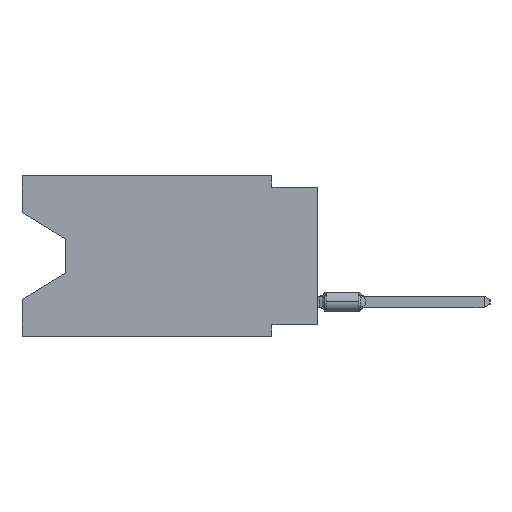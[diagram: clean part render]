
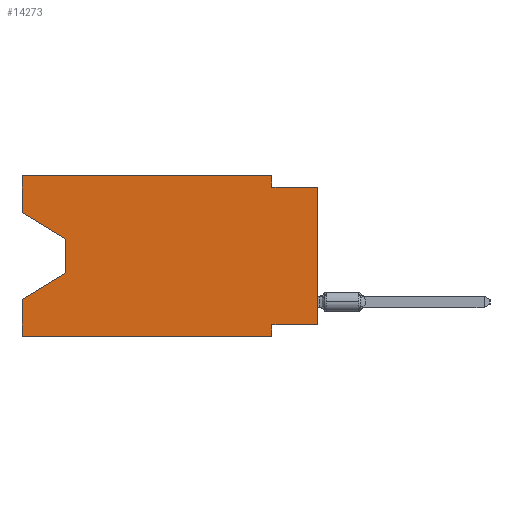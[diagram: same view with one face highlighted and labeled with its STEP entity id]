
A CAD part, left-side view. The second image highlights one B-rep face of the part: STEP entity #14273.
In plain terms, the highlighted planar face has unit normal (-1, 0, 0).
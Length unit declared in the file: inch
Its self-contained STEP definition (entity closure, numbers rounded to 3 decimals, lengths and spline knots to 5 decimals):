
#684 = CARTESIAN_POINT ( 'NONE',  ( 0., 0.645, 0. ) ) ;
#701 = VECTOR ( 'NONE', #1604, 39.37008 ) ;
#1151 = LINE ( 'NONE', #12964, #7756 ) ;
#1463 = EDGE_CURVE ( 'NONE', #5484, #10163, #1151, .T. ) ;
#1604 = DIRECTION ( 'NONE',  ( 0., -1., 0. ) ) ;
#1770 = ORIENTED_EDGE ( 'NONE', *, *, #31686, .F. ) ;
#1779 = DIRECTION ( 'NONE',  ( 0., 0., -1. ) ) ;
#1831 = VERTEX_POINT ( 'NONE', #27846 ) ;
#1860 = FACE_OUTER_BOUND ( 'NONE', #2146, .T. ) ;
#2146 = EDGE_LOOP ( 'NONE', ( #7683, #23044, #23969, #3546, #34981, #1770, #17881, #25467, #27261, #25746, #18919, #8743 ) ) ;
#2795 = VECTOR ( 'NONE', #15203, 39.37008 ) ;
#3060 = VERTEX_POINT ( 'NONE', #7651 ) ;
#3546 = ORIENTED_EDGE ( 'NONE', *, *, #9746, .F. ) ;
#3552 = CARTESIAN_POINT ( 'NONE',  ( 0., 0., -0.325 ) ) ;
#4150 = CARTESIAN_POINT ( 'NONE',  ( 0., 0.55, -0.138 ) ) ;
#4724 = CARTESIAN_POINT ( 'NONE',  ( 0., 0.645, -0.08025 ) ) ;
#5278 = CARTESIAN_POINT ( 'NONE',  ( 0., 0.1, 0. ) ) ;
#5484 = VERTEX_POINT ( 'NONE', #6493 ) ;
#6407 = EDGE_CURVE ( 'NONE', #21673, #17458, #6776, .T. ) ;
#6493 = CARTESIAN_POINT ( 'NONE',  ( 0., 0.645, 0. ) ) ;
#6745 = CARTESIAN_POINT ( 'NONE',  ( 0., 0.1, -0.35 ) ) ;
#6776 = LINE ( 'NONE', #18377, #36574 ) ;
#7187 = LINE ( 'NONE', #34100, #22652 ) ;
#7419 = CARTESIAN_POINT ( 'NONE',  ( 0., 0., -0.025 ) ) ;
#7461 = VERTEX_POINT ( 'NONE', #4724 ) ;
#7474 = PLANE ( 'NONE',  #12363 ) ;
#7651 = CARTESIAN_POINT ( 'NONE',  ( 0., 0.645, -0.35 ) ) ;
#7683 = ORIENTED_EDGE ( 'NONE', *, *, #23505, .T. ) ;
#7756 = VECTOR ( 'NONE', #36549, 39.37008 ) ;
#8116 = CARTESIAN_POINT ( 'NONE',  ( 0., 0.55, -0.138 ) ) ;
#8607 = VERTEX_POINT ( 'NONE', #4150 ) ;
#8667 = EDGE_CURVE ( 'NONE', #3060, #23966, #19072, .T. ) ;
#8743 = ORIENTED_EDGE ( 'NONE', *, *, #22856, .F. ) ;
#9105 = VECTOR ( 'NONE', #21374, 39.37008 ) ;
#9387 = DIRECTION ( 'NONE',  ( 0., 0., 1. ) ) ;
#9746 = EDGE_CURVE ( 'NONE', #3060, #17458, #10046, .T. ) ;
#10046 = LINE ( 'NONE', #21852, #18898 ) ;
#10163 = VERTEX_POINT ( 'NONE', #5278 ) ;
#10171 = DIRECTION ( 'NONE',  ( 1., 0., 0. ) ) ;
#11405 = LINE ( 'NONE', #8116, #35694 ) ;
#12300 = LINE ( 'NONE', #684, #28951 ) ;
#12363 = AXIS2_PLACEMENT_3D ( 'NONE', #19284, #10171, #13275 ) ;
#12964 = CARTESIAN_POINT ( 'NONE',  ( 0., 0.645, 0. ) ) ;
#13275 = DIRECTION ( 'NONE',  ( 0., 0., -1. ) ) ;
#13342 = DIRECTION ( 'NONE',  ( 0., -0.855, -0.519 ) ) ;
#13909 = LINE ( 'NONE', #16812, #34516 ) ;
#14273 = ADVANCED_FACE ( 'NONE', ( #1860 ), #7474, .F. ) ;
#14809 = LINE ( 'NONE', #24293, #31483 ) ;
#15203 = DIRECTION ( 'NONE',  ( 0., -1., 0. ) ) ;
#15305 = CARTESIAN_POINT ( 'NONE',  ( 0., 0.645, -0.26975 ) ) ;
#16230 = CARTESIAN_POINT ( 'NONE',  ( 0., 0., -0.025 ) ) ;
#16812 = CARTESIAN_POINT ( 'NONE',  ( 0., 0.645, -0.08025 ) ) ;
#17161 = EDGE_CURVE ( 'NONE', #1831, #17976, #27742, .T. ) ;
#17403 = CARTESIAN_POINT ( 'NONE',  ( 0., 0.55, -0.212 ) ) ;
#17458 = VERTEX_POINT ( 'NONE', #15305 ) ;
#17881 = ORIENTED_EDGE ( 'NONE', *, *, #35083, .F. ) ;
#17976 = VERTEX_POINT ( 'NONE', #16230 ) ;
#18377 = CARTESIAN_POINT ( 'NONE',  ( 0., 0.55, -0.212 ) ) ;
#18898 = VECTOR ( 'NONE', #33636, 39.37008 ) ;
#18919 = ORIENTED_EDGE ( 'NONE', *, *, #1463, .F. ) ;
#19072 = LINE ( 'NONE', #30870, #2795 ) ;
#19284 = CARTESIAN_POINT ( 'NONE',  ( 0., 0.645, 0. ) ) ;
#20554 = VERTEX_POINT ( 'NONE', #32668 ) ;
#21374 = DIRECTION ( 'NONE',  ( 0., 1., 0. ) ) ;
#21673 = VERTEX_POINT ( 'NONE', #17403 ) ;
#21852 = CARTESIAN_POINT ( 'NONE',  ( 0., 0.645, 0. ) ) ;
#22652 = VECTOR ( 'NONE', #1779, 39.37008 ) ;
#22856 = EDGE_CURVE ( 'NONE', #7461, #5484, #12300, .T. ) ;
#23044 = ORIENTED_EDGE ( 'NONE', *, *, #33446, .T. ) ;
#23505 = EDGE_CURVE ( 'NONE', #7461, #8607, #13909, .T. ) ;
#23921 = DIRECTION ( 'NONE',  ( 0., 0., 1. ) ) ;
#23966 = VERTEX_POINT ( 'NONE', #6745 ) ;
#23969 = ORIENTED_EDGE ( 'NONE', *, *, #6407, .T. ) ;
#24293 = CARTESIAN_POINT ( 'NONE',  ( 0., 0., 0. ) ) ;
#25467 = ORIENTED_EDGE ( 'NONE', *, *, #37052, .T. ) ;
#25746 = ORIENTED_EDGE ( 'NONE', *, *, #30778, .F. ) ;
#27261 = ORIENTED_EDGE ( 'NONE', *, *, #17161, .F. ) ;
#27742 = LINE ( 'NONE', #7419, #701 ) ;
#27846 = CARTESIAN_POINT ( 'NONE',  ( 0., 0.1, -0.025 ) ) ;
#28951 = VECTOR ( 'NONE', #23921, 39.37008 ) ;
#29361 = LINE ( 'NONE', #34961, #29796 ) ;
#29796 = VECTOR ( 'NONE', #38240, 39.37008 ) ;
#30778 = EDGE_CURVE ( 'NONE', #10163, #1831, #29361, .T. ) ;
#30870 = CARTESIAN_POINT ( 'NONE',  ( 0., 0.645, -0.35 ) ) ;
#31483 = VECTOR ( 'NONE', #9387, 39.37008 ) ;
#31686 = EDGE_CURVE ( 'NONE', #20554, #23966, #7187, .T. ) ;
#32668 = CARTESIAN_POINT ( 'NONE',  ( 0., 0.1, -0.325 ) ) ;
#33165 = LINE ( 'NONE', #3552, #9105 ) ;
#33446 = EDGE_CURVE ( 'NONE', #8607, #21673, #11405, .T. ) ;
#33636 = DIRECTION ( 'NONE',  ( 0., 0., 1. ) ) ;
#33866 = DIRECTION ( 'NONE',  ( 0., 0.855, -0.519 ) ) ;
#33963 = VERTEX_POINT ( 'NONE', #34691 ) ;
#34100 = CARTESIAN_POINT ( 'NONE',  ( 0., 0.1, -0.35 ) ) ;
#34516 = VECTOR ( 'NONE', #13342, 39.37008 ) ;
#34691 = CARTESIAN_POINT ( 'NONE',  ( 0., 0., -0.325 ) ) ;
#34961 = CARTESIAN_POINT ( 'NONE',  ( 0., 0.1, 0. ) ) ;
#34981 = ORIENTED_EDGE ( 'NONE', *, *, #8667, .T. ) ;
#34989 = DIRECTION ( 'NONE',  ( 0., 0., -1. ) ) ;
#35083 = EDGE_CURVE ( 'NONE', #33963, #20554, #33165, .T. ) ;
#35694 = VECTOR ( 'NONE', #34989, 39.37008 ) ;
#36549 = DIRECTION ( 'NONE',  ( 0., -1., 0. ) ) ;
#36574 = VECTOR ( 'NONE', #33866, 39.37008 ) ;
#37052 = EDGE_CURVE ( 'NONE', #33963, #17976, #14809, .T. ) ;
#38240 = DIRECTION ( 'NONE',  ( 0., 0., -1. ) ) ;
